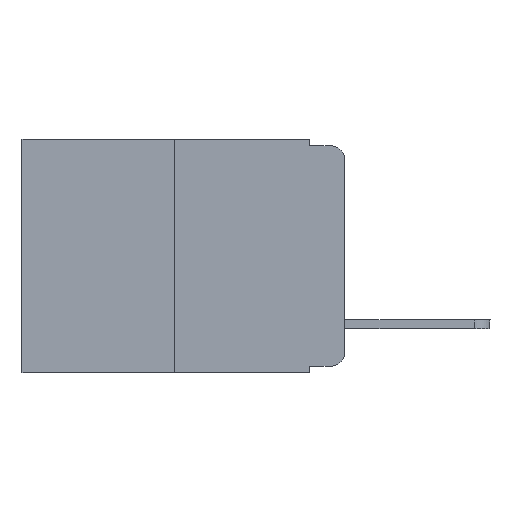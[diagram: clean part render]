
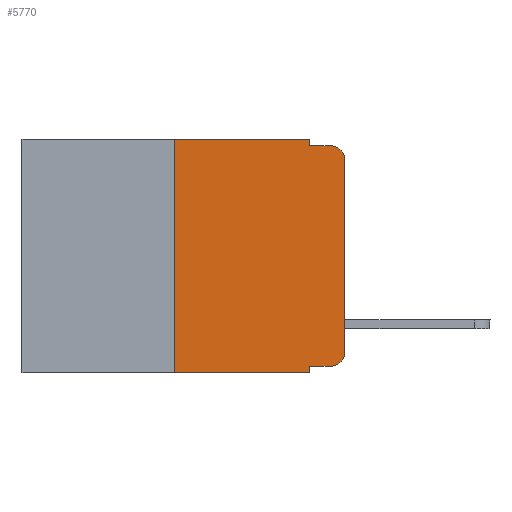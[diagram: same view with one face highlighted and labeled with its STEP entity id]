
A CAD part, left-side view. The second image highlights one B-rep face of the part: STEP entity #5770.
In plain terms, the highlighted planar face has unit normal (-1, 0, 0).
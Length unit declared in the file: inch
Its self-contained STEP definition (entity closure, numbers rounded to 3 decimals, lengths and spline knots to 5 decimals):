
#543 = CARTESIAN_POINT ( 'NONE',  ( 0., 0.051, -0.01 ) ) ;
#666 = VERTEX_POINT ( 'NONE', #9359 ) ;
#676 = DIRECTION ( 'NONE',  ( 0., 0., -1. ) ) ;
#678 = VERTEX_POINT ( 'NONE', #7979 ) ;
#790 = CARTESIAN_POINT ( 'NONE',  ( 0., 0.051, -0.333 ) ) ;
#1341 = CARTESIAN_POINT ( 'NONE',  ( 0., 0.02, -0.01 ) ) ;
#1398 = ORIENTED_EDGE ( 'NONE', *, *, #17624, .T. ) ;
#1896 = CARTESIAN_POINT ( 'NONE',  ( 0., 0., -0.313 ) ) ;
#1942 = VERTEX_POINT ( 'NONE', #5361 ) ;
#2418 = ORIENTED_EDGE ( 'NONE', *, *, #13562, .T. ) ;
#2485 = DIRECTION ( 'NONE',  ( 0., 0., -1. ) ) ;
#2948 = CARTESIAN_POINT ( 'NONE',  ( 0., 0.473, 0. ) ) ;
#3229 = DIRECTION ( 'NONE',  ( 0., -1., 0. ) ) ;
#3533 = CARTESIAN_POINT ( 'NONE',  ( 0., 0., -0.03 ) ) ;
#4704 = VECTOR ( 'NONE', #19064, 39.37008 ) ;
#4751 = EDGE_CURVE ( 'NONE', #1942, #13842, #8229, .T. ) ;
#4831 = VECTOR ( 'NONE', #12208, 39.37008 ) ;
#4922 = VERTEX_POINT ( 'NONE', #543 ) ;
#5270 = LINE ( 'NONE', #14960, #18028 ) ;
#5325 = EDGE_CURVE ( 'NONE', #4922, #18294, #8438, .T. ) ;
#5340 = CARTESIAN_POINT ( 'NONE',  ( 0., 0.051, 0. ) ) ;
#5361 = CARTESIAN_POINT ( 'NONE',  ( 0., 0.051, -0.333 ) ) ;
#5770 = ADVANCED_FACE ( 'NONE', ( #16529 ), #10519, .F. ) ;
#5833 = CIRCLE ( 'NONE', #12892, 0.02 ) ;
#6536 = VERTEX_POINT ( 'NONE', #3533 ) ;
#6557 = EDGE_CURVE ( 'NONE', #666, #13842, #13431, .T. ) ;
#6897 = CARTESIAN_POINT ( 'NONE',  ( 0., 0.02, -0.03 ) ) ;
#6932 = DIRECTION ( 'NONE',  ( -1., 0., 0. ) ) ;
#7050 = EDGE_CURVE ( 'NONE', #678, #16482, #8460, .T. ) ;
#7190 = ORIENTED_EDGE ( 'NONE', *, *, #10738, .F. ) ;
#7268 = VECTOR ( 'NONE', #13852, 39.37008 ) ;
#7764 = ORIENTED_EDGE ( 'NONE', *, *, #9901, .T. ) ;
#7833 = CARTESIAN_POINT ( 'NONE',  ( 0., 0.02, -0.333 ) ) ;
#7979 = CARTESIAN_POINT ( 'NONE',  ( 0., 0.25, 0. ) ) ;
#8229 = LINE ( 'NONE', #13972, #8456 ) ;
#8438 = LINE ( 'NONE', #9296, #18784 ) ;
#8456 = VECTOR ( 'NONE', #13914, 39.37008 ) ;
#8460 = LINE ( 'NONE', #12336, #7268 ) ;
#8770 = CARTESIAN_POINT ( 'NONE',  ( 0., 0.051, -0.343 ) ) ;
#8898 = ORIENTED_EDGE ( 'NONE', *, *, #5325, .F. ) ;
#9296 = CARTESIAN_POINT ( 'NONE',  ( 0., 0.051, -0.01 ) ) ;
#9359 = CARTESIAN_POINT ( 'NONE',  ( 0., 0.25, -0.343 ) ) ;
#9406 = CARTESIAN_POINT ( 'NONE',  ( 0., 0.473, -0.343 ) ) ;
#9434 = VECTOR ( 'NONE', #13992, 39.37008 ) ;
#9842 = CARTESIAN_POINT ( 'NONE',  ( 0., 0.051, 0. ) ) ;
#9901 = EDGE_CURVE ( 'NONE', #19175, #6536, #19243, .T. ) ;
#10519 = PLANE ( 'NONE',  #11170 ) ;
#10651 = LINE ( 'NONE', #790, #4704 ) ;
#10738 = EDGE_CURVE ( 'NONE', #666, #678, #5270, .T. ) ;
#11170 = AXIS2_PLACEMENT_3D ( 'NONE', #2948, #12102, #14868 ) ;
#11324 = LINE ( 'NONE', #9842, #16969 ) ;
#11587 = DIRECTION ( 'NONE',  ( -1., 0., 0. ) ) ;
#11818 = ORIENTED_EDGE ( 'NONE', *, *, #6557, .T. ) ;
#12102 = DIRECTION ( 'NONE',  ( 1., 0., 0. ) ) ;
#12208 = DIRECTION ( 'NONE',  ( 0., 0., 1. ) ) ;
#12336 = CARTESIAN_POINT ( 'NONE',  ( 0., 0.473, 0. ) ) ;
#12673 = EDGE_CURVE ( 'NONE', #16482, #4922, #11324, .T. ) ;
#12731 = ORIENTED_EDGE ( 'NONE', *, *, #4751, .F. ) ;
#12892 = AXIS2_PLACEMENT_3D ( 'NONE', #17375, #6932, #676 ) ;
#13229 = AXIS2_PLACEMENT_3D ( 'NONE', #6897, #11587, #2485 ) ;
#13431 = LINE ( 'NONE', #9406, #9434 ) ;
#13562 = EDGE_CURVE ( 'NONE', #13981, #19175, #5833, .T. ) ;
#13842 = VERTEX_POINT ( 'NONE', #8770 ) ;
#13852 = DIRECTION ( 'NONE',  ( 0., -1., 0. ) ) ;
#13914 = DIRECTION ( 'NONE',  ( 0., 0., -1. ) ) ;
#13972 = CARTESIAN_POINT ( 'NONE',  ( 0., 0.051, 0. ) ) ;
#13981 = VERTEX_POINT ( 'NONE', #7833 ) ;
#13992 = DIRECTION ( 'NONE',  ( 0., -1., 0. ) ) ;
#14868 = DIRECTION ( 'NONE',  ( 0., 0., -1. ) ) ;
#14925 = CIRCLE ( 'NONE', #13229, 0.02 ) ;
#14960 = CARTESIAN_POINT ( 'NONE',  ( 0., 0.25, 0. ) ) ;
#15438 = ORIENTED_EDGE ( 'NONE', *, *, #7050, .F. ) ;
#16064 = DIRECTION ( 'NONE',  ( 0., 0., -1. ) ) ;
#16133 = ORIENTED_EDGE ( 'NONE', *, *, #18728, .T. ) ;
#16482 = VERTEX_POINT ( 'NONE', #5340 ) ;
#16529 = FACE_OUTER_BOUND ( 'NONE', #16836, .T. ) ;
#16777 = CARTESIAN_POINT ( 'NONE',  ( 0., 0., 0. ) ) ;
#16836 = EDGE_LOOP ( 'NONE', ( #7764, #1398, #8898, #19140, #15438, #7190, #11818, #12731, #16133, #2418 ) ) ;
#16969 = VECTOR ( 'NONE', #16064, 39.37008 ) ;
#17375 = CARTESIAN_POINT ( 'NONE',  ( 0., 0.02, -0.313 ) ) ;
#17624 = EDGE_CURVE ( 'NONE', #6536, #18294, #14925, .T. ) ;
#17847 = DIRECTION ( 'NONE',  ( 0., 0., 1. ) ) ;
#18028 = VECTOR ( 'NONE', #17847, 39.37008 ) ;
#18294 = VERTEX_POINT ( 'NONE', #1341 ) ;
#18728 = EDGE_CURVE ( 'NONE', #1942, #13981, #10651, .T. ) ;
#18784 = VECTOR ( 'NONE', #3229, 39.37008 ) ;
#19064 = DIRECTION ( 'NONE',  ( 0., -1., 0. ) ) ;
#19140 = ORIENTED_EDGE ( 'NONE', *, *, #12673, .F. ) ;
#19175 = VERTEX_POINT ( 'NONE', #1896 ) ;
#19243 = LINE ( 'NONE', #16777, #4831 ) ;
